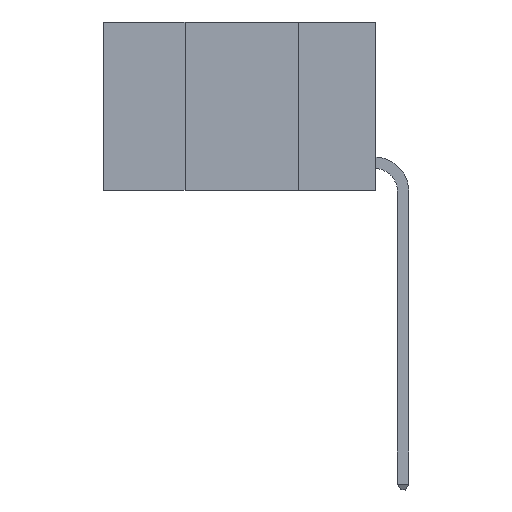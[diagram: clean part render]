
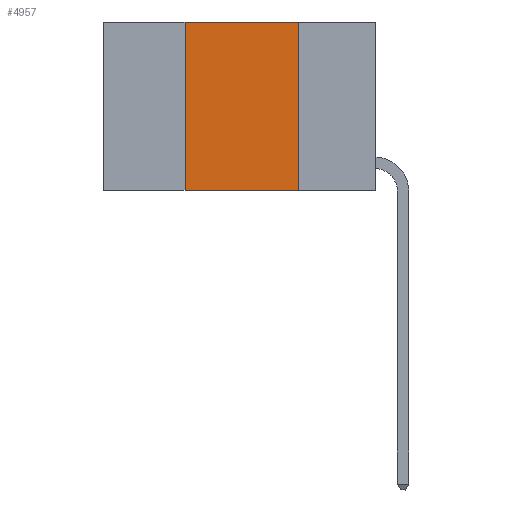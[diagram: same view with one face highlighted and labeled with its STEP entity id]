
A CAD part, left-side view. The second image highlights one B-rep face of the part: STEP entity #4957.
In plain terms, the highlighted planar face has unit normal (-1, 0, 0).
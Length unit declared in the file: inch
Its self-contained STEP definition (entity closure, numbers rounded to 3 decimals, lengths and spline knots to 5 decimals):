
#166 = LINE ( 'NONE', #4741, #14981 ) ;
#1619 = LINE ( 'NONE', #9385, #5038 ) ;
#2288 = ORIENTED_EDGE ( 'NONE', *, *, #12119, .T. ) ;
#2607 = FACE_OUTER_BOUND ( 'NONE', #5855, .T. ) ;
#2933 = EDGE_CURVE ( 'NONE', #5925, #2967, #9940, .T. ) ;
#2967 = VERTEX_POINT ( 'NONE', #11626 ) ;
#3028 = PLANE ( 'NONE',  #17240 ) ;
#3085 = DIRECTION ( 'NONE',  ( 0., 0., -1. ) ) ;
#3438 = DIRECTION ( 'NONE',  ( 0., 0., -1. ) ) ;
#4741 = CARTESIAN_POINT ( 'NONE',  ( 0., 0.42, 0. ) ) ;
#4957 = ADVANCED_FACE ( 'NONE', ( #2607 ), #3028, .F. ) ;
#5038 = VECTOR ( 'NONE', #10800, 39.37008 ) ;
#5065 = EDGE_CURVE ( 'NONE', #15734, #5925, #166, .T. ) ;
#5235 = ORIENTED_EDGE ( 'NONE', *, *, #14612, .F. ) ;
#5487 = CARTESIAN_POINT ( 'NONE',  ( 0., 0.42, 0. ) ) ;
#5855 = EDGE_LOOP ( 'NONE', ( #5235, #13278, #17029, #2288 ) ) ;
#5925 = VERTEX_POINT ( 'NONE', #5487 ) ;
#6880 = CARTESIAN_POINT ( 'NONE',  ( 0., 0.17, -0.37 ) ) ;
#7905 = VECTOR ( 'NONE', #3438, 39.37008 ) ;
#7921 = CARTESIAN_POINT ( 'NONE',  ( 0., 0.42, -0.37 ) ) ;
#9385 = CARTESIAN_POINT ( 'NONE',  ( 0., 0.6, -0.37 ) ) ;
#9490 = VECTOR ( 'NONE', #13799, 39.37008 ) ;
#9940 = LINE ( 'NONE', #16143, #9490 ) ;
#10800 = DIRECTION ( 'NONE',  ( 0., -1., 0. ) ) ;
#11626 = CARTESIAN_POINT ( 'NONE',  ( 0., 0.17, 0. ) ) ;
#11677 = DIRECTION ( 'NONE',  ( 1., 0., 0. ) ) ;
#12119 = EDGE_CURVE ( 'NONE', #15734, #16613, #1619, .T. ) ;
#12121 = LINE ( 'NONE', #13497, #7905 ) ;
#13278 = ORIENTED_EDGE ( 'NONE', *, *, #2933, .F. ) ;
#13497 = CARTESIAN_POINT ( 'NONE',  ( 0., 0.17, 0. ) ) ;
#13799 = DIRECTION ( 'NONE',  ( 0., -1., 0. ) ) ;
#14612 = EDGE_CURVE ( 'NONE', #2967, #16613, #12121, .T. ) ;
#14981 = VECTOR ( 'NONE', #16170, 39.37008 ) ;
#15734 = VERTEX_POINT ( 'NONE', #7921 ) ;
#15920 = CARTESIAN_POINT ( 'NONE',  ( 0., 0.6, 0. ) ) ;
#16143 = CARTESIAN_POINT ( 'NONE',  ( 0., 0.6, 0. ) ) ;
#16170 = DIRECTION ( 'NONE',  ( 0., 0., 1. ) ) ;
#16613 = VERTEX_POINT ( 'NONE', #6880 ) ;
#17029 = ORIENTED_EDGE ( 'NONE', *, *, #5065, .F. ) ;
#17240 = AXIS2_PLACEMENT_3D ( 'NONE', #15920, #11677, #3085 ) ;
